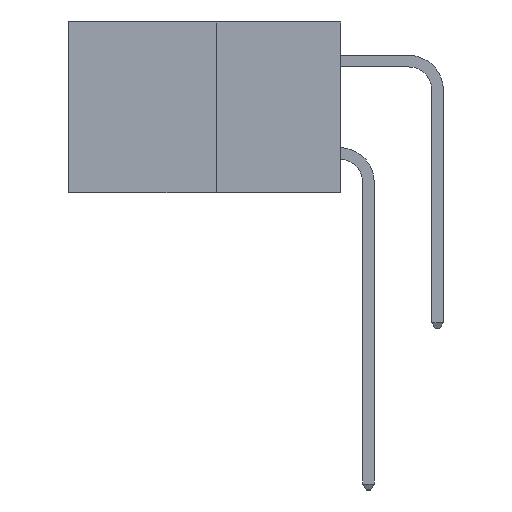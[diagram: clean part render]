
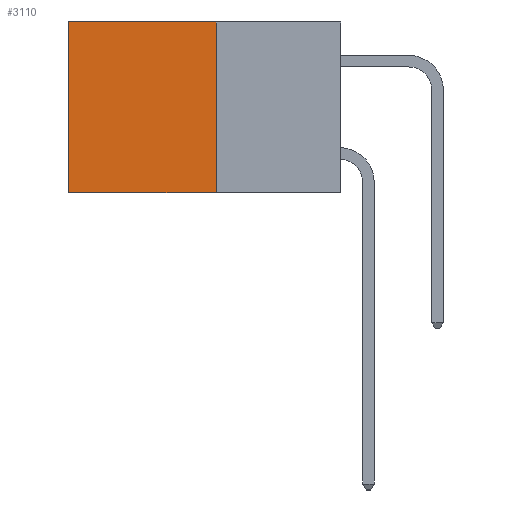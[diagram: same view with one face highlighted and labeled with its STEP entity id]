
A CAD part, left-side view. The second image highlights one B-rep face of the part: STEP entity #3110.
In plain terms, the highlighted planar face has unit normal (-1, 0, 0).
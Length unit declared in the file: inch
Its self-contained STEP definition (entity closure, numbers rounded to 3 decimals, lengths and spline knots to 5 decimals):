
#34 = DIRECTION ( 'NONE',  ( 0., 0., -1. ) ) ;
#316 = VECTOR ( 'NONE', #34, 39.37008 ) ;
#529 = CARTESIAN_POINT ( 'NONE',  ( 0.277, 0.59, -0.37 ) ) ;
#685 = VERTEX_POINT ( 'NONE', #3923 ) ;
#869 = FACE_OUTER_BOUND ( 'NONE', #5442, .T. ) ;
#1150 = EDGE_CURVE ( 'NONE', #685, #1457, #5422, .T. ) ;
#1317 = ORIENTED_EDGE ( 'NONE', *, *, #9473, .T. ) ;
#1328 = DIRECTION ( 'NONE',  ( 0., 1., 0. ) ) ;
#1419 = VECTOR ( 'NONE', #8624, 39.37008 ) ;
#1457 = VERTEX_POINT ( 'NONE', #529 ) ;
#1557 = EDGE_CURVE ( 'NONE', #1558, #685, #4357, .T. ) ;
#1558 = VERTEX_POINT ( 'NONE', #6412 ) ;
#2218 = ORIENTED_EDGE ( 'NONE', *, *, #7418, .T. ) ;
#2731 = DIRECTION ( 'NONE',  ( 0., 0., -1. ) ) ;
#3110 = ADVANCED_FACE ( 'NONE', ( #869 ), #7589, .F. ) ;
#3713 = AXIS2_PLACEMENT_3D ( 'NONE', #8355, #5126, #6956 ) ;
#3923 = CARTESIAN_POINT ( 'NONE',  ( 0.277, 0.27, -0.37 ) ) ;
#4357 = LINE ( 'NONE', #7906, #316 ) ;
#4920 = CARTESIAN_POINT ( 'NONE',  ( 0.277, 0.27, -0.37 ) ) ;
#5080 = CARTESIAN_POINT ( 'NONE',  ( 0.277, 0.27, 0. ) ) ;
#5126 = DIRECTION ( 'NONE',  ( 1., 0., 0. ) ) ;
#5150 = LINE ( 'NONE', #5080, #8834 ) ;
#5422 = LINE ( 'NONE', #4920, #1419 ) ;
#5442 = EDGE_LOOP ( 'NONE', ( #2218, #5976, #8229, #1317 ) ) ;
#5543 = VECTOR ( 'NONE', #2731, 39.37008 ) ;
#5711 = CARTESIAN_POINT ( 'NONE',  ( 0.277, 0.59, -0.37 ) ) ;
#5976 = ORIENTED_EDGE ( 'NONE', *, *, #1150, .F. ) ;
#6412 = CARTESIAN_POINT ( 'NONE',  ( 0.277, 0.27, 0. ) ) ;
#6956 = DIRECTION ( 'NONE',  ( 0., 0., -1. ) ) ;
#7178 = VERTEX_POINT ( 'NONE', #8414 ) ;
#7418 = EDGE_CURVE ( 'NONE', #7178, #1457, #9657, .T. ) ;
#7589 = PLANE ( 'NONE',  #3713 ) ;
#7906 = CARTESIAN_POINT ( 'NONE',  ( 0.277, 0.27, -0.37 ) ) ;
#8229 = ORIENTED_EDGE ( 'NONE', *, *, #1557, .F. ) ;
#8355 = CARTESIAN_POINT ( 'NONE',  ( 0.277, 0.27, -0.37 ) ) ;
#8414 = CARTESIAN_POINT ( 'NONE',  ( 0.277, 0.59, 0. ) ) ;
#8624 = DIRECTION ( 'NONE',  ( 0., 1., 0. ) ) ;
#8834 = VECTOR ( 'NONE', #1328, 39.37008 ) ;
#9473 = EDGE_CURVE ( 'NONE', #1558, #7178, #5150, .T. ) ;
#9657 = LINE ( 'NONE', #5711, #5543 ) ;
